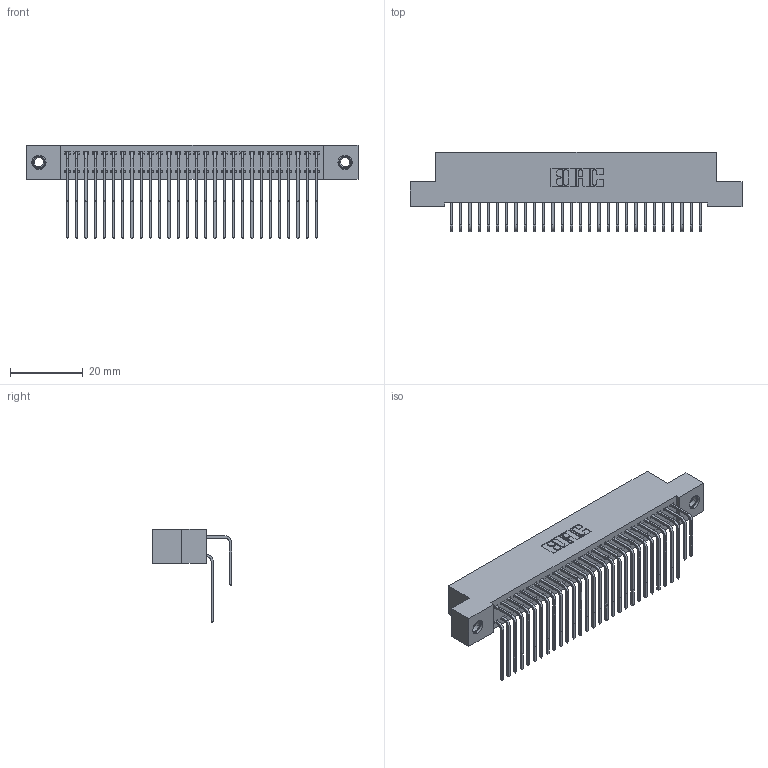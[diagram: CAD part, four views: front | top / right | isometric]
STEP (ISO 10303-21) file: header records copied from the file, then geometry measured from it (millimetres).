
FILE_DESCRIPTION (( 'STEP AP203' ), '1' );
FILE_NAME ('342-056-558-207.STEP', '2019-10-03T11:44:11', ( '' ), ( '' ), 'SwSTEP 2.0', 'SolidWorks 2016', '' );
FILE_SCHEMA (( 'CONFIG_CONTROL_DESIGN' ));
Length unit declared in the file: inch
Products named in the file (5): 345-292-001_558 559 Tail - 1; 345-292-001_558 Tail - 2; 345-250-001_345-250-005-103; 342-056-558-207; 342 Part_TI
Assembly tree (59 placements, depth 2):
  342-056-558-207
    342 Part_TI
    345-292-001_558 559 Tail - 1  x28
    345-292-001_558 Tail - 2  x28
    345-250-001_345-250-005-103  x2
Bounding box: 91.44 x 21.91 x 25.78 mm (x, y, z)
Volume: 8460 mm3; surface area: 14912.9 mm2
Topology: 59 solids, 59 shells, 3194 faces, 9451 edges, 6218 vertices
Faces by surface type: plane 2226, cylinder 952, cone 12, torus 4
Entity records: 22662 total; most frequent: CARTESIAN_POINT 3804, ORIENTED_EDGE 3682, DIRECTION 3287, EDGE_CURVE 1841, LINE 1653, VECTOR 1653, VERTEX_POINT 1220, AXIS2_PLACEMENT_3D 817
